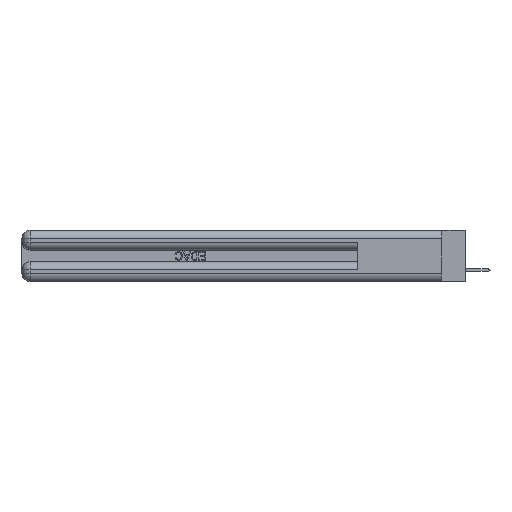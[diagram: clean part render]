
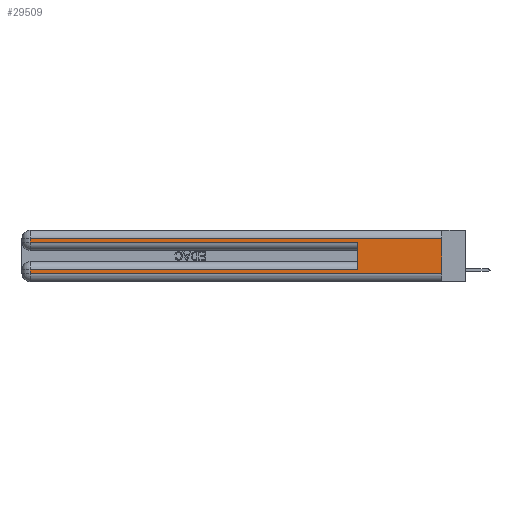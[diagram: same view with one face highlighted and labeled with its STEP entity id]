
A CAD part, left-side view. The second image highlights one B-rep face of the part: STEP entity #29509.
In plain terms, the highlighted planar face has unit normal (-1, 0, 0).
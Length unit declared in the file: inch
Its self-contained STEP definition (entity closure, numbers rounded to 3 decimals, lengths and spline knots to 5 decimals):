
#550 = DIRECTION ( 'NONE',  ( 0., 0., -1. ) ) ;
#758 = DIRECTION ( 'NONE',  ( 0., 1., 0. ) ) ;
#1305 = VERTEX_POINT ( 'NONE', #12365 ) ;
#2329 = CARTESIAN_POINT ( 'NONE',  ( 0., 0., 0.37 ) ) ;
#3570 = LINE ( 'NONE', #6367, #46425 ) ;
#4360 = VECTOR ( 'NONE', #46798, 39.37008 ) ;
#5406 = LINE ( 'NONE', #47643, #43397 ) ;
#5857 = VECTOR ( 'NONE', #49678, 39.37008 ) ;
#6270 = CARTESIAN_POINT ( 'NONE',  ( 0., 0., 0.085 ) ) ;
#6367 = CARTESIAN_POINT ( 'NONE',  ( 0., 2.94, 0.37 ) ) ;
#7502 = EDGE_CURVE ( 'NONE', #28883, #9233, #19394, .T. ) ;
#7881 = LINE ( 'NONE', #11836, #14582 ) ;
#9233 = VERTEX_POINT ( 'NONE', #36339 ) ;
#10180 = DIRECTION ( 'NONE',  ( 1., 0., 0. ) ) ;
#11383 = ORIENTED_EDGE ( 'NONE', *, *, #23386, .F. ) ;
#11836 = CARTESIAN_POINT ( 'NONE',  ( 0., 0., 0.37 ) ) ;
#12365 = CARTESIAN_POINT ( 'NONE',  ( 0., 2.94, 0.06 ) ) ;
#12419 = EDGE_CURVE ( 'NONE', #1305, #49925, #32693, .T. ) ;
#13282 = ORIENTED_EDGE ( 'NONE', *, *, #42993, .F. ) ;
#14056 = VERTEX_POINT ( 'NONE', #43102 ) ;
#14582 = VECTOR ( 'NONE', #23847, 39.37008 ) ;
#16176 = ORIENTED_EDGE ( 'NONE', *, *, #28790, .T. ) ;
#16242 = FACE_OUTER_BOUND ( 'NONE', #34127, .T. ) ;
#18815 = ORIENTED_EDGE ( 'NONE', *, *, #20988, .T. ) ;
#19301 = VERTEX_POINT ( 'NONE', #28524 ) ;
#19394 = LINE ( 'NONE', #27420, #36592 ) ;
#20109 = DIRECTION ( 'NONE',  ( 0., 0., 1. ) ) ;
#20370 = AXIS2_PLACEMENT_3D ( 'NONE', #2329, #10180, #45289 ) ;
#20988 = EDGE_CURVE ( 'NONE', #14056, #19301, #31280, .T. ) ;
#23081 = ORIENTED_EDGE ( 'NONE', *, *, #43363, .T. ) ;
#23386 = EDGE_CURVE ( 'NONE', #43404, #19301, #5406, .T. ) ;
#23847 = DIRECTION ( 'NONE',  ( 0., 0., -1. ) ) ;
#23936 = CARTESIAN_POINT ( 'NONE',  ( 0., 0., 0.06 ) ) ;
#24308 = VECTOR ( 'NONE', #550, 39.37008 ) ;
#24694 = VECTOR ( 'NONE', #34721, 39.37008 ) ;
#26011 = CARTESIAN_POINT ( 'NONE',  ( 0., 0., 0.31 ) ) ;
#26183 = ORIENTED_EDGE ( 'NONE', *, *, #7502, .T. ) ;
#26907 = ORIENTED_EDGE ( 'NONE', *, *, #29529, .T. ) ;
#27210 = VERTEX_POINT ( 'NONE', #46758 ) ;
#27420 = CARTESIAN_POINT ( 'NONE',  ( 0., 0., 0.31 ) ) ;
#27984 = LINE ( 'NONE', #43512, #24308 ) ;
#28524 = CARTESIAN_POINT ( 'NONE',  ( 0., 0.6, 0.285 ) ) ;
#28790 = EDGE_CURVE ( 'NONE', #27210, #1305, #27984, .T. ) ;
#28883 = VERTEX_POINT ( 'NONE', #26011 ) ;
#29509 = ADVANCED_FACE ( 'NONE', ( #16242 ), #41385, .F. ) ;
#29529 = EDGE_CURVE ( 'NONE', #43404, #27210, #48055, .T. ) ;
#31280 = LINE ( 'NONE', #34655, #4360 ) ;
#32693 = LINE ( 'NONE', #49910, #24694 ) ;
#34127 = EDGE_LOOP ( 'NONE', ( #13282, #26183, #23081, #18815, #11383, #26907, #16176, #34435 ) ) ;
#34435 = ORIENTED_EDGE ( 'NONE', *, *, #12419, .T. ) ;
#34655 = CARTESIAN_POINT ( 'NONE',  ( 0., 0., 0.285 ) ) ;
#34721 = DIRECTION ( 'NONE',  ( 0., -1., 0. ) ) ;
#36339 = CARTESIAN_POINT ( 'NONE',  ( 0., 2.94, 0.31 ) ) ;
#36592 = VECTOR ( 'NONE', #758, 39.37008 ) ;
#37518 = CARTESIAN_POINT ( 'NONE',  ( 0., 0.6, 0.085 ) ) ;
#37847 = DIRECTION ( 'NONE',  ( 0., 0., -1. ) ) ;
#41385 = PLANE ( 'NONE',  #20370 ) ;
#42993 = EDGE_CURVE ( 'NONE', #28883, #49925, #7881, .T. ) ;
#43102 = CARTESIAN_POINT ( 'NONE',  ( 0., 2.94, 0.285 ) ) ;
#43363 = EDGE_CURVE ( 'NONE', #9233, #14056, #3570, .T. ) ;
#43397 = VECTOR ( 'NONE', #20109, 39.37008 ) ;
#43404 = VERTEX_POINT ( 'NONE', #37518 ) ;
#43512 = CARTESIAN_POINT ( 'NONE',  ( 0., 2.94, 0.37 ) ) ;
#45289 = DIRECTION ( 'NONE',  ( 0., 0., -1. ) ) ;
#46425 = VECTOR ( 'NONE', #37847, 39.37008 ) ;
#46758 = CARTESIAN_POINT ( 'NONE',  ( 0., 2.94, 0.085 ) ) ;
#46798 = DIRECTION ( 'NONE',  ( 0., -1., 0. ) ) ;
#47643 = CARTESIAN_POINT ( 'NONE',  ( 0., 0.6, 0.145 ) ) ;
#48055 = LINE ( 'NONE', #6270, #5857 ) ;
#49678 = DIRECTION ( 'NONE',  ( 0., 1., 0. ) ) ;
#49910 = CARTESIAN_POINT ( 'NONE',  ( 0., 0., 0.06 ) ) ;
#49925 = VERTEX_POINT ( 'NONE', #23936 ) ;
